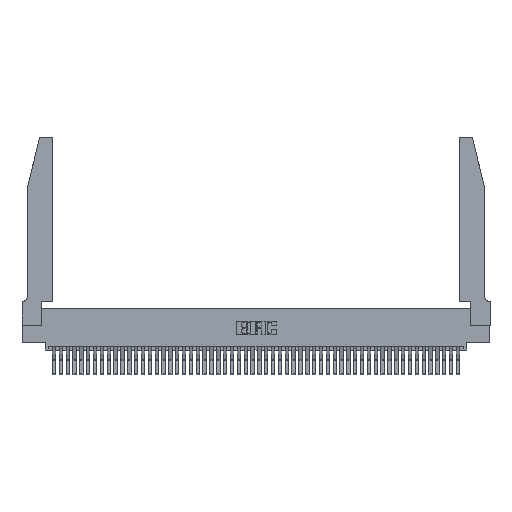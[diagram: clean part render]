
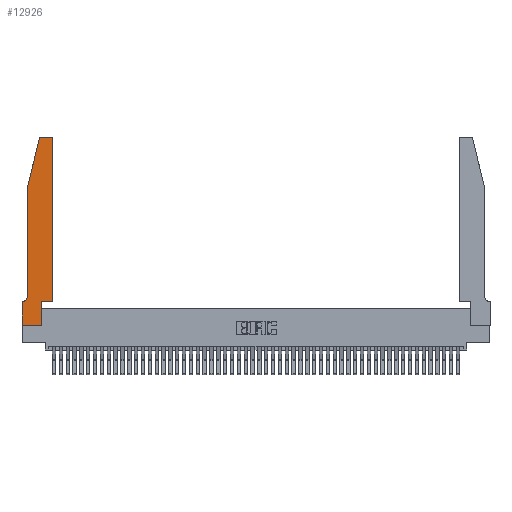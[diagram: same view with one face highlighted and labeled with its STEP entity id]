
A CAD part, top view. The second image highlights one B-rep face of the part: STEP entity #12926.
In plain terms, the highlighted planar face has unit normal (0, 0, 1).
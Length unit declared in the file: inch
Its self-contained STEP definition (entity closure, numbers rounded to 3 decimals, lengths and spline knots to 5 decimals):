
#2042 = EDGE_CURVE ( 'NONE', #44070, #32417, #23946, .T. ) ;
#2134 = EDGE_CURVE ( 'NONE', #11477, #47200, #40654, .T. ) ;
#2315 = CARTESIAN_POINT ( 'NONE',  ( 0.284, 2.72, 0.37 ) ) ;
#3041 = DIRECTION ( 'NONE',  ( 0., 0., 1. ) ) ;
#3077 = ORIENTED_EDGE ( 'NONE', *, *, #6984, .T. ) ;
#3182 = CARTESIAN_POINT ( 'NONE',  ( 0., 0., 0.37 ) ) ;
#3554 = ORIENTED_EDGE ( 'NONE', *, *, #2042, .T. ) ;
#4065 = CARTESIAN_POINT ( 'NONE',  ( 0., 0., 0.37 ) ) ;
#4576 = CARTESIAN_POINT ( 'NONE',  ( 0.0755, 2., 0.37 ) ) ;
#4946 = ORIENTED_EDGE ( 'NONE', *, *, #44495, .T. ) ;
#5275 = EDGE_CURVE ( 'NONE', #28480, #10126, #45073, .T. ) ;
#5653 = LINE ( 'NONE', #10934, #46401 ) ;
#6042 = LINE ( 'NONE', #14991, #35449 ) ;
#6164 = DIRECTION ( 'NONE',  ( 1., 0., 0. ) ) ;
#6399 = CIRCLE ( 'NONE', #44730, 0.03 ) ;
#6572 = LINE ( 'NONE', #41566, #25892 ) ;
#6984 = EDGE_CURVE ( 'NONE', #22891, #9522, #19423, .T. ) ;
#7128 = ORIENTED_EDGE ( 'NONE', *, *, #23609, .T. ) ;
#8528 = ORIENTED_EDGE ( 'NONE', *, *, #21090, .T. ) ;
#8924 = AXIS2_PLACEMENT_3D ( 'NONE', #26131, #3041, #29956 ) ;
#9522 = VERTEX_POINT ( 'NONE', #30372 ) ;
#10012 = VECTOR ( 'NONE', #19635, 39.37008 ) ;
#10126 = VERTEX_POINT ( 'NONE', #18267 ) ;
#10564 = CARTESIAN_POINT ( 'NONE',  ( 0.4205, 2.75, 0.37 ) ) ;
#10934 = CARTESIAN_POINT ( 'NONE',  ( 0.4505, 0.35, 0.37 ) ) ;
#11077 = DIRECTION ( 'NONE',  ( 0., 1., 0. ) ) ;
#11477 = VERTEX_POINT ( 'NONE', #31991 ) ;
#11605 = EDGE_LOOP ( 'NONE', ( #7128, #33876, #33652, #8528, #3077, #22781, #3554, #37152, #13927, #37810, #18943, #4946 ) ) ;
#12447 = EDGE_CURVE ( 'NONE', #9522, #44070, #6572, .T. ) ;
#12906 = DIRECTION ( 'NONE',  ( -0.239, -0.971, 0. ) ) ;
#12926 = ADVANCED_FACE ( 'NONE', ( #27039 ), #33699, .T. ) ;
#13827 = EDGE_CURVE ( 'NONE', #32417, #21662, #29334, .T. ) ;
#13927 = ORIENTED_EDGE ( 'NONE', *, *, #35213, .T. ) ;
#14595 = DIRECTION ( 'NONE',  ( 0., 0., 1. ) ) ;
#14991 = CARTESIAN_POINT ( 'NONE',  ( 0.2865, 0.35, 0.37 ) ) ;
#15354 = CARTESIAN_POINT ( 'NONE',  ( 0.2865, 0., 0.37 ) ) ;
#15588 = CARTESIAN_POINT ( 'NONE',  ( 0., 0., 0.37 ) ) ;
#18224 = VECTOR ( 'NONE', #47949, 39.37008 ) ;
#18267 = CARTESIAN_POINT ( 'NONE',  ( 0.4505, 2.72, 0.37 ) ) ;
#18801 = CARTESIAN_POINT ( 'NONE',  ( 0.0755, 0.42, 0.37 ) ) ;
#18943 = ORIENTED_EDGE ( 'NONE', *, *, #5275, .T. ) ;
#19134 = VECTOR ( 'NONE', #12906, 39.37008 ) ;
#19423 = CIRCLE ( 'NONE', #24564, 0.07 ) ;
#19490 = DIRECTION ( 'NONE',  ( 0., -1., 0. ) ) ;
#19635 = DIRECTION ( 'NONE',  ( 0., -1., 0. ) ) ;
#20427 = CARTESIAN_POINT ( 'NONE',  ( 0.2865, 0.35, 0.37 ) ) ;
#20479 = CIRCLE ( 'NONE', #8924, 0.03 ) ;
#20545 = DIRECTION ( 'NONE',  ( 0., 1., 0. ) ) ;
#21090 = EDGE_CURVE ( 'NONE', #47200, #22891, #30480, .T. ) ;
#21662 = VERTEX_POINT ( 'NONE', #15354 ) ;
#22756 = VECTOR ( 'NONE', #19490, 39.37008 ) ;
#22781 = ORIENTED_EDGE ( 'NONE', *, *, #12447, .T. ) ;
#22891 = VERTEX_POINT ( 'NONE', #18801 ) ;
#22930 = CARTESIAN_POINT ( 'NONE',  ( 0.0055, 0.42, 0.37 ) ) ;
#23177 = VERTEX_POINT ( 'NONE', #20427 ) ;
#23609 = EDGE_CURVE ( 'NONE', #24470, #29883, #29620, .T. ) ;
#23620 = VECTOR ( 'NONE', #20545, 39.37008 ) ;
#23849 = CARTESIAN_POINT ( 'NONE',  ( 0.4505, 0.35, 0.37 ) ) ;
#23946 = LINE ( 'NONE', #15588, #22756 ) ;
#24470 = VERTEX_POINT ( 'NONE', #10564 ) ;
#24564 = AXIS2_PLACEMENT_3D ( 'NONE', #22930, #49583, #26779 ) ;
#25892 = VECTOR ( 'NONE', #45391, 39.37008 ) ;
#26131 = CARTESIAN_POINT ( 'NONE',  ( 0.4205, 2.72, 0.37 ) ) ;
#26779 = DIRECTION ( 'NONE',  ( -1., 0., 0. ) ) ;
#27039 = FACE_OUTER_BOUND ( 'NONE', #11605, .T. ) ;
#27673 = CARTESIAN_POINT ( 'NONE',  ( 0., 0.35, 0.37 ) ) ;
#28480 = VERTEX_POINT ( 'NONE', #23849 ) ;
#29227 = DIRECTION ( 'NONE',  ( 0., 0., 1. ) ) ;
#29334 = LINE ( 'NONE', #4065, #49590 ) ;
#29620 = LINE ( 'NONE', #44116, #18224 ) ;
#29883 = VERTEX_POINT ( 'NONE', #37626 ) ;
#29956 = DIRECTION ( 'NONE',  ( 1., 0., 0. ) ) ;
#30280 = DIRECTION ( 'NONE',  ( 1., 0., 0. ) ) ;
#30372 = CARTESIAN_POINT ( 'NONE',  ( 0.0055, 0.35, 0.37 ) ) ;
#30480 = LINE ( 'NONE', #38647, #10012 ) ;
#30961 = DIRECTION ( 'NONE',  ( 1., 0., 0. ) ) ;
#31914 = CARTESIAN_POINT ( 'NONE',  ( 0.4505, 0.35, 0.37 ) ) ;
#31991 = CARTESIAN_POINT ( 'NONE',  ( 0.25487, 2.72718, 0.37 ) ) ;
#32417 = VERTEX_POINT ( 'NONE', #3182 ) ;
#33312 = EDGE_CURVE ( 'NONE', #23177, #28480, #5653, .T. ) ;
#33652 = ORIENTED_EDGE ( 'NONE', *, *, #2134, .T. ) ;
#33699 = PLANE ( 'NONE',  #36507 ) ;
#33876 = ORIENTED_EDGE ( 'NONE', *, *, #39012, .T. ) ;
#35213 = EDGE_CURVE ( 'NONE', #21662, #23177, #6042, .T. ) ;
#35449 = VECTOR ( 'NONE', #11077, 39.37008 ) ;
#36507 = AXIS2_PLACEMENT_3D ( 'NONE', #37519, #14595, #41378 ) ;
#37152 = ORIENTED_EDGE ( 'NONE', *, *, #13827, .T. ) ;
#37519 = CARTESIAN_POINT ( 'NONE',  ( 0., 0.35, 0.37 ) ) ;
#37626 = CARTESIAN_POINT ( 'NONE',  ( 0.284, 2.75, 0.37 ) ) ;
#37810 = ORIENTED_EDGE ( 'NONE', *, *, #33312, .T. ) ;
#38647 = CARTESIAN_POINT ( 'NONE',  ( 0.0755, 2., 0.37 ) ) ;
#39012 = EDGE_CURVE ( 'NONE', #29883, #11477, #6399, .T. ) ;
#39523 = CARTESIAN_POINT ( 'NONE',  ( 0.0755, 2., 0.37 ) ) ;
#40654 = LINE ( 'NONE', #39523, #19134 ) ;
#41378 = DIRECTION ( 'NONE',  ( 1., 0., 0. ) ) ;
#41566 = CARTESIAN_POINT ( 'NONE',  ( 0.0755, 0.35, 0.37 ) ) ;
#44070 = VERTEX_POINT ( 'NONE', #27673 ) ;
#44116 = CARTESIAN_POINT ( 'NONE',  ( 0.2605, 2.75, 0.37 ) ) ;
#44495 = EDGE_CURVE ( 'NONE', #10126, #24470, #20479, .T. ) ;
#44730 = AXIS2_PLACEMENT_3D ( 'NONE', #2315, #29227, #6164 ) ;
#45073 = LINE ( 'NONE', #31914, #23620 ) ;
#45391 = DIRECTION ( 'NONE',  ( -1., 0., 0. ) ) ;
#46401 = VECTOR ( 'NONE', #30280, 39.37008 ) ;
#47200 = VERTEX_POINT ( 'NONE', #4576 ) ;
#47949 = DIRECTION ( 'NONE',  ( -1., 0., 0. ) ) ;
#49583 = DIRECTION ( 'NONE',  ( 0., 0., -1. ) ) ;
#49590 = VECTOR ( 'NONE', #30961, 39.37008 ) ;
